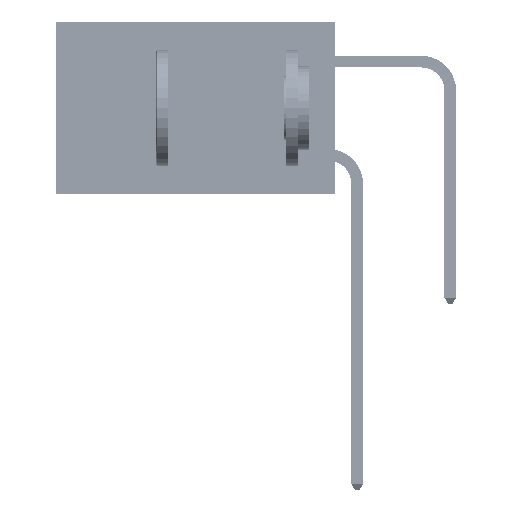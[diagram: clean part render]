
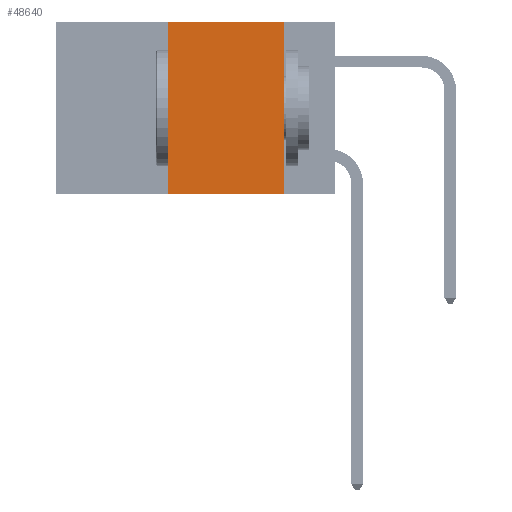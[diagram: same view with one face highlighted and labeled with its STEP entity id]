
A CAD part, left-side view. The second image highlights one B-rep face of the part: STEP entity #48640.
In plain terms, the highlighted planar face has unit normal (-1, 0, 0).
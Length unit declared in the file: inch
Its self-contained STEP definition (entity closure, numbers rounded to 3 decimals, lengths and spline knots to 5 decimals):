
#546 = VERTEX_POINT ( 'NONE', #19525 ) ;
#1081 = VERTEX_POINT ( 'NONE', #2623 ) ;
#1620 = VERTEX_POINT ( 'NONE', #37971 ) ;
#1996 = CARTESIAN_POINT ( 'NONE',  ( 0., 0.6, 0. ) ) ;
#2623 = CARTESIAN_POINT ( 'NONE',  ( 0., 0.36, -0.37 ) ) ;
#5846 = LINE ( 'NONE', #48540, #47719 ) ;
#5907 = EDGE_CURVE ( 'NONE', #1081, #9351, #41751, .T. ) ;
#6029 = DIRECTION ( 'NONE',  ( 0., 0., -1. ) ) ;
#9063 = ORIENTED_EDGE ( 'NONE', *, *, #28953, .F. ) ;
#9236 = VECTOR ( 'NONE', #19778, 39.37008 ) ;
#9351 = VERTEX_POINT ( 'NONE', #47522 ) ;
#10330 = ORIENTED_EDGE ( 'NONE', *, *, #5907, .F. ) ;
#10391 = VECTOR ( 'NONE', #20033, 39.37008 ) ;
#11951 = EDGE_CURVE ( 'NONE', #1081, #546, #5846, .T. ) ;
#15818 = CARTESIAN_POINT ( 'NONE',  ( 0., 0.6, 0. ) ) ;
#18293 = AXIS2_PLACEMENT_3D ( 'NONE', #1996, #29675, #6029 ) ;
#19525 = CARTESIAN_POINT ( 'NONE',  ( 0., 0.11, -0.37 ) ) ;
#19559 = LINE ( 'NONE', #38009, #49595 ) ;
#19778 = DIRECTION ( 'NONE',  ( 0., -1., 0. ) ) ;
#20033 = DIRECTION ( 'NONE',  ( 0., 0., 1. ) ) ;
#21768 = PLANE ( 'NONE',  #18293 ) ;
#23301 = ORIENTED_EDGE ( 'NONE', *, *, #11951, .T. ) ;
#23408 = EDGE_CURVE ( 'NONE', #1620, #546, #19559, .T. ) ;
#28953 = EDGE_CURVE ( 'NONE', #9351, #1620, #40610, .T. ) ;
#29012 = DIRECTION ( 'NONE',  ( 0., -1., 0. ) ) ;
#29675 = DIRECTION ( 'NONE',  ( 1., 0., 0. ) ) ;
#35142 = FACE_OUTER_BOUND ( 'NONE', #47131, .T. ) ;
#36774 = ORIENTED_EDGE ( 'NONE', *, *, #23408, .F. ) ;
#37971 = CARTESIAN_POINT ( 'NONE',  ( 0., 0.11, 0. ) ) ;
#38009 = CARTESIAN_POINT ( 'NONE',  ( 0., 0.11, 0. ) ) ;
#40610 = LINE ( 'NONE', #15818, #9236 ) ;
#41751 = LINE ( 'NONE', #47471, #10391 ) ;
#41938 = DIRECTION ( 'NONE',  ( 0., 0., -1. ) ) ;
#47131 = EDGE_LOOP ( 'NONE', ( #36774, #9063, #10330, #23301 ) ) ;
#47471 = CARTESIAN_POINT ( 'NONE',  ( 0., 0.36, 0. ) ) ;
#47522 = CARTESIAN_POINT ( 'NONE',  ( 0., 0.36, 0. ) ) ;
#47719 = VECTOR ( 'NONE', #29012, 39.37008 ) ;
#48540 = CARTESIAN_POINT ( 'NONE',  ( 0., 0.6, -0.37 ) ) ;
#48640 = ADVANCED_FACE ( 'NONE', ( #35142 ), #21768, .F. ) ;
#49595 = VECTOR ( 'NONE', #41938, 39.37008 ) ;
